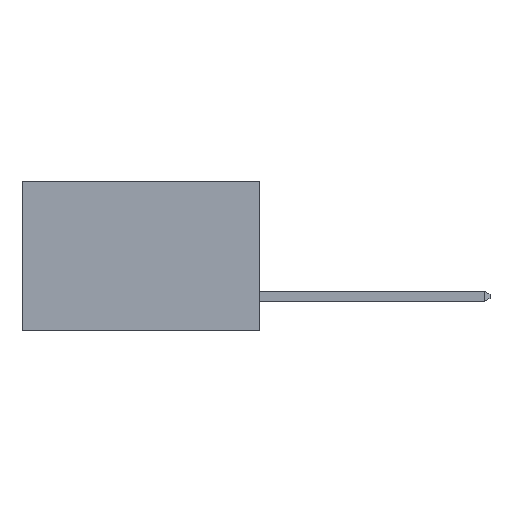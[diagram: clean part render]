
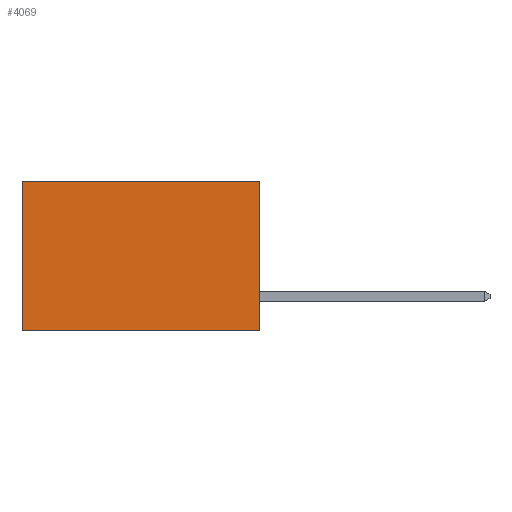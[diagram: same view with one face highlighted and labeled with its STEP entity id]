
A CAD part, left-side view. The second image highlights one B-rep face of the part: STEP entity #4069.
In plain terms, the highlighted planar face has unit normal (-1, 0, 0).
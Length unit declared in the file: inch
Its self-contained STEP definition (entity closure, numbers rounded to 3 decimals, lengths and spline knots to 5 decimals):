
#63 = FACE_OUTER_BOUND ( 'NONE', #2078, .T. ) ;
#149 = LINE ( 'NONE', #509, #10499 ) ;
#484 = AXIS2_PLACEMENT_3D ( 'NONE', #7367, #4281, #9708 ) ;
#509 = CARTESIAN_POINT ( 'NONE',  ( 0.277, 0.59, -0.37 ) ) ;
#713 = DIRECTION ( 'NONE',  ( 0., 1., 0. ) ) ;
#1136 = CARTESIAN_POINT ( 'NONE',  ( 0.277, 0.59, 0. ) ) ;
#1674 = CARTESIAN_POINT ( 'NONE',  ( 0.277, 0., 0. ) ) ;
#2078 = EDGE_LOOP ( 'NONE', ( #4692, #5042, #5894, #7272 ) ) ;
#3253 = VERTEX_POINT ( 'NONE', #7569 ) ;
#3677 = DIRECTION ( 'NONE',  ( 0., 1., 0. ) ) ;
#4069 = ADVANCED_FACE ( 'NONE', ( #63 ), #5886, .F. ) ;
#4281 = DIRECTION ( 'NONE',  ( 1., 0., 0. ) ) ;
#4301 = EDGE_CURVE ( 'NONE', #3253, #12068, #8049, .T. ) ;
#4692 = ORIENTED_EDGE ( 'NONE', *, *, #10033, .T. ) ;
#4888 = VECTOR ( 'NONE', #7083, 39.37008 ) ;
#5042 = ORIENTED_EDGE ( 'NONE', *, *, #4301, .F. ) ;
#5886 = PLANE ( 'NONE',  #484 ) ;
#5894 = ORIENTED_EDGE ( 'NONE', *, *, #9147, .F. ) ;
#6494 = EDGE_CURVE ( 'NONE', #7285, #7069, #8305, .T. ) ;
#6668 = CARTESIAN_POINT ( 'NONE',  ( 0.277, 0.59, -0.37 ) ) ;
#7069 = VERTEX_POINT ( 'NONE', #1136 ) ;
#7083 = DIRECTION ( 'NONE',  ( 0., 0., -1. ) ) ;
#7272 = ORIENTED_EDGE ( 'NONE', *, *, #6494, .T. ) ;
#7285 = VERTEX_POINT ( 'NONE', #11017 ) ;
#7367 = CARTESIAN_POINT ( 'NONE',  ( 0.277, 0., -0.37 ) ) ;
#7569 = CARTESIAN_POINT ( 'NONE',  ( 0.277, 0., -0.37 ) ) ;
#7997 = VECTOR ( 'NONE', #713, 39.37008 ) ;
#8049 = LINE ( 'NONE', #12436, #12679 ) ;
#8305 = LINE ( 'NONE', #1674, #7997 ) ;
#9147 = EDGE_CURVE ( 'NONE', #7285, #3253, #11898, .T. ) ;
#9708 = DIRECTION ( 'NONE',  ( 0., 0., -1. ) ) ;
#10033 = EDGE_CURVE ( 'NONE', #7069, #12068, #149, .T. ) ;
#10499 = VECTOR ( 'NONE', #11417, 39.37008 ) ;
#11017 = CARTESIAN_POINT ( 'NONE',  ( 0.277, 0., 0. ) ) ;
#11417 = DIRECTION ( 'NONE',  ( 0., 0., -1. ) ) ;
#11898 = LINE ( 'NONE', #12699, #4888 ) ;
#12068 = VERTEX_POINT ( 'NONE', #6668 ) ;
#12436 = CARTESIAN_POINT ( 'NONE',  ( 0.277, 0., -0.37 ) ) ;
#12679 = VECTOR ( 'NONE', #3677, 39.37008 ) ;
#12699 = CARTESIAN_POINT ( 'NONE',  ( 0.277, 0., -0.37 ) ) ;
